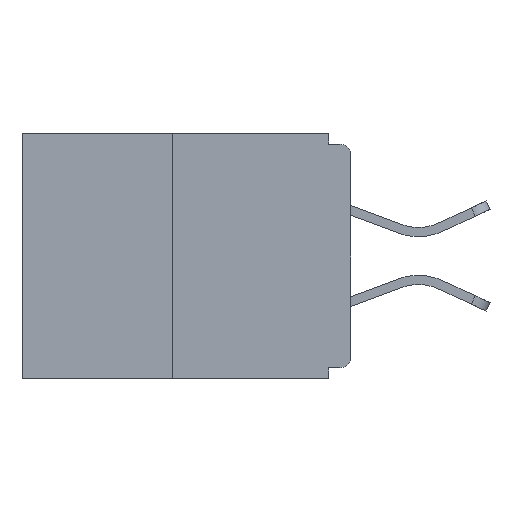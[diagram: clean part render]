
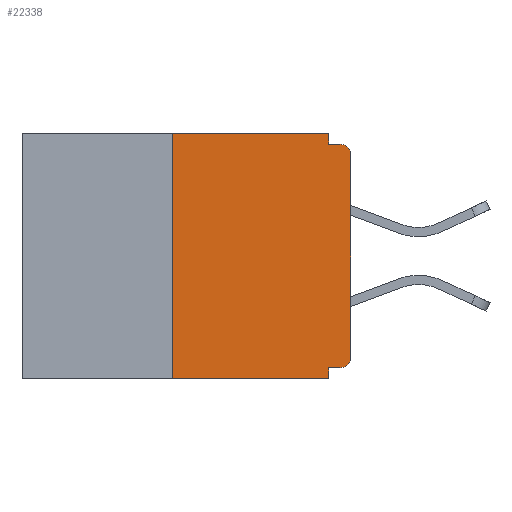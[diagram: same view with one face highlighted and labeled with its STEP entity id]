
A CAD part, left-side view. The second image highlights one B-rep face of the part: STEP entity #22338.
In plain terms, the highlighted planar face has unit normal (-1, 0, 0).
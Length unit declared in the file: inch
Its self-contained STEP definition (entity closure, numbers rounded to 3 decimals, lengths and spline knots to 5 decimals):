
#359 = VERTEX_POINT ( 'NONE', #8748 ) ;
#793 = PLANE ( 'NONE',  #14211 ) ;
#919 = CARTESIAN_POINT ( 'NONE',  ( 0., 0., -0.328 ) ) ;
#1269 = LINE ( 'NONE', #919, #24712 ) ;
#3060 = EDGE_CURVE ( 'NONE', #359, #24591, #16211, .T. ) ;
#3266 = ORIENTED_EDGE ( 'NONE', *, *, #21777, .T. ) ;
#3303 = CARTESIAN_POINT ( 'NONE',  ( 0., 0.031, -0.015 ) ) ;
#3386 = VECTOR ( 'NONE', #13072, 39.37008 ) ;
#3675 = EDGE_CURVE ( 'NONE', #20058, #13555, #5871, .T. ) ;
#4016 = CARTESIAN_POINT ( 'NONE',  ( 0., 0.25, 0. ) ) ;
#4253 = CARTESIAN_POINT ( 'NONE',  ( 0., 0., -0.313 ) ) ;
#5871 = LINE ( 'NONE', #13768, #13587 ) ;
#5893 = ORIENTED_EDGE ( 'NONE', *, *, #13446, .F. ) ;
#6295 = EDGE_CURVE ( 'NONE', #12185, #9464, #30059, .T. ) ;
#6979 = AXIS2_PLACEMENT_3D ( 'NONE', #29256, #26591, #12749 ) ;
#7432 = LINE ( 'NONE', #4016, #3386 ) ;
#7644 = ORIENTED_EDGE ( 'NONE', *, *, #10027, .F. ) ;
#8748 = CARTESIAN_POINT ( 'NONE',  ( 0., 0.031, -0.328 ) ) ;
#9435 = VECTOR ( 'NONE', #26544, 39.37008 ) ;
#9464 = VERTEX_POINT ( 'NONE', #4253 ) ;
#10027 = EDGE_CURVE ( 'NONE', #12185, #359, #1269, .T. ) ;
#10151 = DIRECTION ( 'NONE',  ( 0., 0., -1. ) ) ;
#10487 = LINE ( 'NONE', #22128, #12293 ) ;
#10864 = AXIS2_PLACEMENT_3D ( 'NONE', #20835, #18309, #22975 ) ;
#12185 = VERTEX_POINT ( 'NONE', #16909 ) ;
#12271 = CARTESIAN_POINT ( 'NONE',  ( 0., 0., -0.03 ) ) ;
#12293 = VECTOR ( 'NONE', #29781, 39.37008 ) ;
#12407 = CARTESIAN_POINT ( 'NONE',  ( 0., 0.031, 0. ) ) ;
#12749 = DIRECTION ( 'NONE',  ( 0., 0., -1. ) ) ;
#12871 = CARTESIAN_POINT ( 'NONE',  ( 0., 0.25, -0.343 ) ) ;
#13072 = DIRECTION ( 'NONE',  ( 0., 0., 1. ) ) ;
#13446 = EDGE_CURVE ( 'NONE', #26553, #27763, #7432, .T. ) ;
#13555 = VERTEX_POINT ( 'NONE', #13581 ) ;
#13581 = CARTESIAN_POINT ( 'NONE',  ( 0., 0.015, -0.015 ) ) ;
#13587 = VECTOR ( 'NONE', #27718, 39.37008 ) ;
#13661 = EDGE_CURVE ( 'NONE', #20774, #13555, #22848, .T. ) ;
#13768 = CARTESIAN_POINT ( 'NONE',  ( 0., 0., -0.015 ) ) ;
#14077 = FACE_OUTER_BOUND ( 'NONE', #22092, .T. ) ;
#14145 = ORIENTED_EDGE ( 'NONE', *, *, #21066, .T. ) ;
#14211 = AXIS2_PLACEMENT_3D ( 'NONE', #29003, #22087, #10151 ) ;
#15969 = LINE ( 'NONE', #29746, #25090 ) ;
#16211 = LINE ( 'NONE', #20239, #23484 ) ;
#16391 = LINE ( 'NONE', #27839, #25847 ) ;
#16909 = CARTESIAN_POINT ( 'NONE',  ( 0., 0.015, -0.328 ) ) ;
#18102 = EDGE_CURVE ( 'NONE', #20243, #20058, #19650, .T. ) ;
#18309 = DIRECTION ( 'NONE',  ( -1., 0., 0. ) ) ;
#19333 = ORIENTED_EDGE ( 'NONE', *, *, #22078, .F. ) ;
#19558 = ORIENTED_EDGE ( 'NONE', *, *, #3675, .F. ) ;
#19650 = LINE ( 'NONE', #24457, #9435 ) ;
#20058 = VERTEX_POINT ( 'NONE', #3303 ) ;
#20079 = ORIENTED_EDGE ( 'NONE', *, *, #6295, .T. ) ;
#20239 = CARTESIAN_POINT ( 'NONE',  ( 0., 0.031, -0.343 ) ) ;
#20243 = VERTEX_POINT ( 'NONE', #12407 ) ;
#20774 = VERTEX_POINT ( 'NONE', #12271 ) ;
#20835 = CARTESIAN_POINT ( 'NONE',  ( 0., 0.015, -0.03 ) ) ;
#21066 = EDGE_CURVE ( 'NONE', #26553, #24591, #16391, .T. ) ;
#21777 = EDGE_CURVE ( 'NONE', #9464, #20774, #10487, .T. ) ;
#22078 = EDGE_CURVE ( 'NONE', #27763, #20243, #15969, .T. ) ;
#22087 = DIRECTION ( 'NONE',  ( 1., 0., 0. ) ) ;
#22092 = EDGE_LOOP ( 'NONE', ( #19333, #5893, #14145, #28601, #7644, #20079, #3266, #23885, #19558, #25458 ) ) ;
#22128 = CARTESIAN_POINT ( 'NONE',  ( 0., 0., 0. ) ) ;
#22338 = ADVANCED_FACE ( 'NONE', ( #14077 ), #793, .F. ) ;
#22578 = DIRECTION ( 'NONE',  ( 0., 0., -1. ) ) ;
#22848 = CIRCLE ( 'NONE', #10864, 0.015 ) ;
#22975 = DIRECTION ( 'NONE',  ( 0., 0., -1. ) ) ;
#23484 = VECTOR ( 'NONE', #22578, 39.37008 ) ;
#23885 = ORIENTED_EDGE ( 'NONE', *, *, #13661, .T. ) ;
#24457 = CARTESIAN_POINT ( 'NONE',  ( 0., 0.031, 0. ) ) ;
#24591 = VERTEX_POINT ( 'NONE', #29139 ) ;
#24673 = DIRECTION ( 'NONE',  ( 0., 1., 0. ) ) ;
#24712 = VECTOR ( 'NONE', #24673, 39.37008 ) ;
#25090 = VECTOR ( 'NONE', #27168, 39.37008 ) ;
#25458 = ORIENTED_EDGE ( 'NONE', *, *, #18102, .F. ) ;
#25847 = VECTOR ( 'NONE', #30317, 39.37008 ) ;
#26544 = DIRECTION ( 'NONE',  ( 0., 0., -1. ) ) ;
#26553 = VERTEX_POINT ( 'NONE', #12871 ) ;
#26591 = DIRECTION ( 'NONE',  ( -1., 0., 0. ) ) ;
#27168 = DIRECTION ( 'NONE',  ( 0., -1., 0. ) ) ;
#27718 = DIRECTION ( 'NONE',  ( 0., -1., 0. ) ) ;
#27763 = VERTEX_POINT ( 'NONE', #29845 ) ;
#27839 = CARTESIAN_POINT ( 'NONE',  ( 0., 0.46, -0.343 ) ) ;
#28601 = ORIENTED_EDGE ( 'NONE', *, *, #3060, .F. ) ;
#29003 = CARTESIAN_POINT ( 'NONE',  ( 0., 0.46, 0. ) ) ;
#29139 = CARTESIAN_POINT ( 'NONE',  ( 0., 0.031, -0.343 ) ) ;
#29256 = CARTESIAN_POINT ( 'NONE',  ( 0., 0.015, -0.313 ) ) ;
#29746 = CARTESIAN_POINT ( 'NONE',  ( 0., 0.46, 0. ) ) ;
#29781 = DIRECTION ( 'NONE',  ( 0., 0., 1. ) ) ;
#29845 = CARTESIAN_POINT ( 'NONE',  ( 0., 0.25, 0. ) ) ;
#30059 = CIRCLE ( 'NONE', #6979, 0.015 ) ;
#30317 = DIRECTION ( 'NONE',  ( 0., -1., 0. ) ) ;
